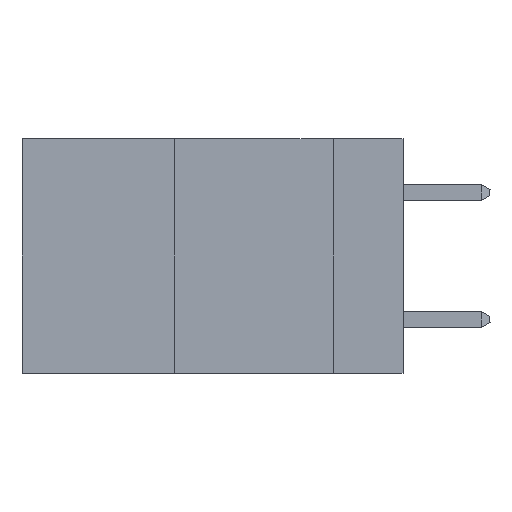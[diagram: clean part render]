
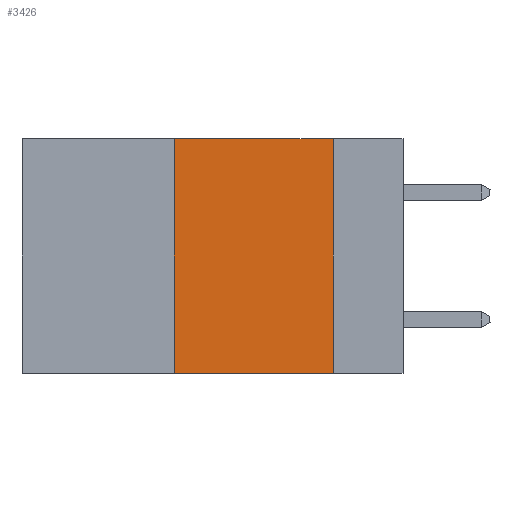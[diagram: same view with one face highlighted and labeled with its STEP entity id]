
A CAD part, left-side view. The second image highlights one B-rep face of the part: STEP entity #3426.
In plain terms, the highlighted planar face has unit normal (-1, 0, 0).
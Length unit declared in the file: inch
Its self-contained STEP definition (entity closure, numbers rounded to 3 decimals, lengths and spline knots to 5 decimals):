
#914 = LINE ( 'NONE', #14408, #34926 ) ;
#1616 = VECTOR ( 'NONE', #34677, 39.37008 ) ;
#2570 = AXIS2_PLACEMENT_3D ( 'NONE', #18522, #7021, #12815 ) ;
#3426 = ADVANCED_FACE ( 'NONE', ( #15356 ), #30066, .F. ) ;
#5476 = LINE ( 'NONE', #36363, #13573 ) ;
#6317 = EDGE_CURVE ( 'NONE', #23794, #27470, #32401, .T. ) ;
#7021 = DIRECTION ( 'NONE',  ( 1., 0., 0. ) ) ;
#8217 = CARTESIAN_POINT ( 'NONE',  ( 0., 0.11, 0. ) ) ;
#8624 = DIRECTION ( 'NONE',  ( 0., -1., 0. ) ) ;
#8656 = CARTESIAN_POINT ( 'NONE',  ( 0., 0.11, -0.37 ) ) ;
#9982 = CARTESIAN_POINT ( 'NONE',  ( 0., 0.11, 0. ) ) ;
#10070 = DIRECTION ( 'NONE',  ( 0., 0., 1. ) ) ;
#12815 = DIRECTION ( 'NONE',  ( 0., 0., -1. ) ) ;
#12963 = CARTESIAN_POINT ( 'NONE',  ( 0., 0.36, 0. ) ) ;
#13261 = VERTEX_POINT ( 'NONE', #30608 ) ;
#13573 = VECTOR ( 'NONE', #33188, 39.37008 ) ;
#13817 = VERTEX_POINT ( 'NONE', #17564 ) ;
#14408 = CARTESIAN_POINT ( 'NONE',  ( 0., 0.6, 0. ) ) ;
#15356 = FACE_OUTER_BOUND ( 'NONE', #24102, .T. ) ;
#17564 = CARTESIAN_POINT ( 'NONE',  ( 0., 0.36, -0.37 ) ) ;
#18522 = CARTESIAN_POINT ( 'NONE',  ( 0., 0.6, 0. ) ) ;
#18539 = ORIENTED_EDGE ( 'NONE', *, *, #25738, .F. ) ;
#19365 = LINE ( 'NONE', #12963, #26130 ) ;
#23794 = VERTEX_POINT ( 'NONE', #9982 ) ;
#24102 = EDGE_LOOP ( 'NONE', ( #31122, #31733, #18539, #30749 ) ) ;
#25738 = EDGE_CURVE ( 'NONE', #13817, #13261, #19365, .T. ) ;
#26130 = VECTOR ( 'NONE', #10070, 39.37008 ) ;
#27470 = VERTEX_POINT ( 'NONE', #8656 ) ;
#30066 = PLANE ( 'NONE',  #2570 ) ;
#30608 = CARTESIAN_POINT ( 'NONE',  ( 0., 0.36, 0. ) ) ;
#30749 = ORIENTED_EDGE ( 'NONE', *, *, #31845, .T. ) ;
#31122 = ORIENTED_EDGE ( 'NONE', *, *, #6317, .F. ) ;
#31733 = ORIENTED_EDGE ( 'NONE', *, *, #36683, .F. ) ;
#31845 = EDGE_CURVE ( 'NONE', #13817, #27470, #5476, .T. ) ;
#32401 = LINE ( 'NONE', #8217, #1616 ) ;
#33188 = DIRECTION ( 'NONE',  ( 0., -1., 0. ) ) ;
#34677 = DIRECTION ( 'NONE',  ( 0., 0., -1. ) ) ;
#34926 = VECTOR ( 'NONE', #8624, 39.37008 ) ;
#36363 = CARTESIAN_POINT ( 'NONE',  ( 0., 0.6, -0.37 ) ) ;
#36683 = EDGE_CURVE ( 'NONE', #13261, #23794, #914, .T. ) ;
